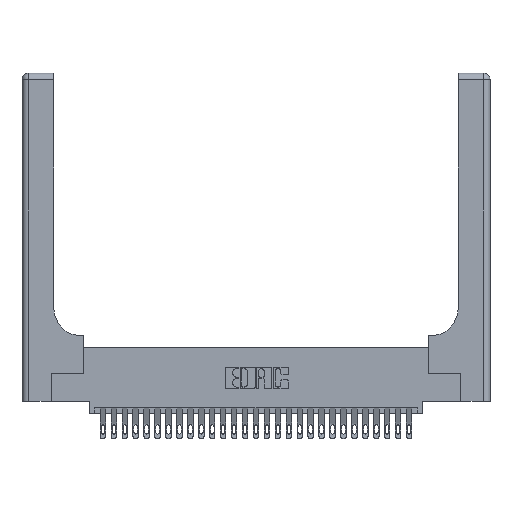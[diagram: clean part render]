
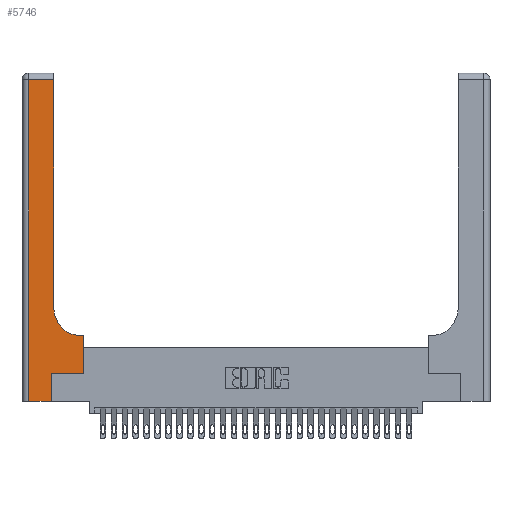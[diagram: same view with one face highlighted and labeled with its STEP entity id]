
A CAD part, top view. The second image highlights one B-rep face of the part: STEP entity #5746.
In plain terms, the highlighted planar face has unit normal (0, 0, 1).
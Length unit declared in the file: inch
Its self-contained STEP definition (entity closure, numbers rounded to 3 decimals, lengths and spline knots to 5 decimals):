
#324 = DIRECTION ( 'NONE',  ( 0., 1., 0. ) ) ;
#1182 = EDGE_LOOP ( 'NONE', ( #10315, #29504, #5516, #12549, #24899, #20244, #2199, #27757, #16953 ) ) ;
#1794 = LINE ( 'NONE', #4662, #14379 ) ;
#2092 = DIRECTION ( 'NONE',  ( 1., 0., 0. ) ) ;
#2199 = ORIENTED_EDGE ( 'NONE', *, *, #18743, .T. ) ;
#3418 = CARTESIAN_POINT ( 'NONE',  ( 0., 3., 0.37 ) ) ;
#3529 = AXIS2_PLACEMENT_3D ( 'NONE', #3418, #10548, #26786 ) ;
#3949 = EDGE_CURVE ( 'NONE', #7037, #27100, #6667, .T. ) ;
#4662 = CARTESIAN_POINT ( 'NONE',  ( 0.2915, 0.6, 0.37 ) ) ;
#5516 = ORIENTED_EDGE ( 'NONE', *, *, #9253, .T. ) ;
#5746 = ADVANCED_FACE ( 'NONE', ( #28008 ), #8164, .F. ) ;
#5961 = EDGE_CURVE ( 'NONE', #29549, #19945, #23022, .T. ) ;
#6577 = EDGE_CURVE ( 'NONE', #19945, #18088, #18662, .T. ) ;
#6667 = LINE ( 'NONE', #22683, #19168 ) ;
#6912 = DIRECTION ( 'NONE',  ( 1., 0., 0. ) ) ;
#7037 = VERTEX_POINT ( 'NONE', #22464 ) ;
#7685 = EDGE_CURVE ( 'NONE', #15648, #24620, #27209, .T. ) ;
#7755 = CARTESIAN_POINT ( 'NONE',  ( 0.06, 3., 0.37 ) ) ;
#8164 = PLANE ( 'NONE',  #3529 ) ;
#9253 = EDGE_CURVE ( 'NONE', #27100, #26299, #13811, .T. ) ;
#9837 = CARTESIAN_POINT ( 'NONE',  ( 0.2915, 3., 0.37 ) ) ;
#10315 = ORIENTED_EDGE ( 'NONE', *, *, #11060, .T. ) ;
#10548 = DIRECTION ( 'NONE',  ( 0., 0., -1. ) ) ;
#11060 = EDGE_CURVE ( 'NONE', #24620, #7037, #17672, .T. ) ;
#11064 = DIRECTION ( 'NONE',  ( -1., 0., 0. ) ) ;
#11534 = LINE ( 'NONE', #27810, #29233 ) ;
#11645 = CARTESIAN_POINT ( 'NONE',  ( 0., 0., 0.37 ) ) ;
#11752 = CARTESIAN_POINT ( 'NONE',  ( 0.5585, 0.25, 0.37 ) ) ;
#11823 = CARTESIAN_POINT ( 'NONE',  ( 0.269, 0., 0.37 ) ) ;
#12407 = VECTOR ( 'NONE', #6912, 39.37008 ) ;
#12549 = ORIENTED_EDGE ( 'NONE', *, *, #16971, .T. ) ;
#12592 = VECTOR ( 'NONE', #14041, 39.37008 ) ;
#13811 = LINE ( 'NONE', #7755, #24659 ) ;
#13859 = CARTESIAN_POINT ( 'NONE',  ( 0.269, 0.25, 0.37 ) ) ;
#14041 = DIRECTION ( 'NONE',  ( 1., 0., 0. ) ) ;
#14379 = VECTOR ( 'NONE', #21116, 39.37008 ) ;
#15243 = AXIS2_PLACEMENT_3D ( 'NONE', #29969, #16220, #2092 ) ;
#15648 = VERTEX_POINT ( 'NONE', #22444 ) ;
#16220 = DIRECTION ( 'NONE',  ( 0., 0., -1. ) ) ;
#16921 = VECTOR ( 'NONE', #324, 39.37008 ) ;
#16953 = ORIENTED_EDGE ( 'NONE', *, *, #7685, .T. ) ;
#16971 = EDGE_CURVE ( 'NONE', #26299, #29549, #18832, .T. ) ;
#16977 = CARTESIAN_POINT ( 'NONE',  ( 0.06, 2.94, 0.37 ) ) ;
#17585 = VECTOR ( 'NONE', #20914, 39.37008 ) ;
#17672 = LINE ( 'NONE', #9837, #16921 ) ;
#18088 = VERTEX_POINT ( 'NONE', #11752 ) ;
#18652 = CARTESIAN_POINT ( 'NONE',  ( 0.269, 0.25, 0.37 ) ) ;
#18662 = LINE ( 'NONE', #18652, #12407 ) ;
#18743 = EDGE_CURVE ( 'NONE', #18088, #29945, #11534, .T. ) ;
#18800 = DIRECTION ( 'NONE',  ( 0., 1., 0. ) ) ;
#18832 = LINE ( 'NONE', #11645, #12592 ) ;
#19168 = VECTOR ( 'NONE', #11064, 39.37008 ) ;
#19945 = VERTEX_POINT ( 'NONE', #13859 ) ;
#20244 = ORIENTED_EDGE ( 'NONE', *, *, #6577, .T. ) ;
#20914 = DIRECTION ( 'NONE',  ( 0., 1., 0. ) ) ;
#21116 = DIRECTION ( 'NONE',  ( -1., 0., 0. ) ) ;
#22444 = CARTESIAN_POINT ( 'NONE',  ( 0.5415, 0.6, 0.37 ) ) ;
#22464 = CARTESIAN_POINT ( 'NONE',  ( 0.2915, 2.94, 0.37 ) ) ;
#22683 = CARTESIAN_POINT ( 'NONE',  ( 0., 2.94, 0.37 ) ) ;
#23022 = LINE ( 'NONE', #27790, #17585 ) ;
#24207 = DIRECTION ( 'NONE',  ( 0., -1., 0. ) ) ;
#24620 = VERTEX_POINT ( 'NONE', #28897 ) ;
#24659 = VECTOR ( 'NONE', #24207, 39.37008 ) ;
#24899 = ORIENTED_EDGE ( 'NONE', *, *, #5961, .T. ) ;
#26299 = VERTEX_POINT ( 'NONE', #29566 ) ;
#26786 = DIRECTION ( 'NONE',  ( -1., 0., 0. ) ) ;
#26903 = CARTESIAN_POINT ( 'NONE',  ( 0.5585, 0.6, 0.37 ) ) ;
#27100 = VERTEX_POINT ( 'NONE', #16977 ) ;
#27209 = CIRCLE ( 'NONE', #15243, 0.25 ) ;
#27757 = ORIENTED_EDGE ( 'NONE', *, *, #28280, .T. ) ;
#27790 = CARTESIAN_POINT ( 'NONE',  ( 0.269, 0., 0.37 ) ) ;
#27810 = CARTESIAN_POINT ( 'NONE',  ( 0.5585, 0.25, 0.37 ) ) ;
#28008 = FACE_OUTER_BOUND ( 'NONE', #1182, .T. ) ;
#28280 = EDGE_CURVE ( 'NONE', #29945, #15648, #1794, .T. ) ;
#28897 = CARTESIAN_POINT ( 'NONE',  ( 0.2915, 0.85, 0.37 ) ) ;
#29233 = VECTOR ( 'NONE', #18800, 39.37008 ) ;
#29504 = ORIENTED_EDGE ( 'NONE', *, *, #3949, .T. ) ;
#29549 = VERTEX_POINT ( 'NONE', #11823 ) ;
#29566 = CARTESIAN_POINT ( 'NONE',  ( 0.06, 0., 0.37 ) ) ;
#29945 = VERTEX_POINT ( 'NONE', #26903 ) ;
#29969 = CARTESIAN_POINT ( 'NONE',  ( 0.5415, 0.85, 0.37 ) ) ;
